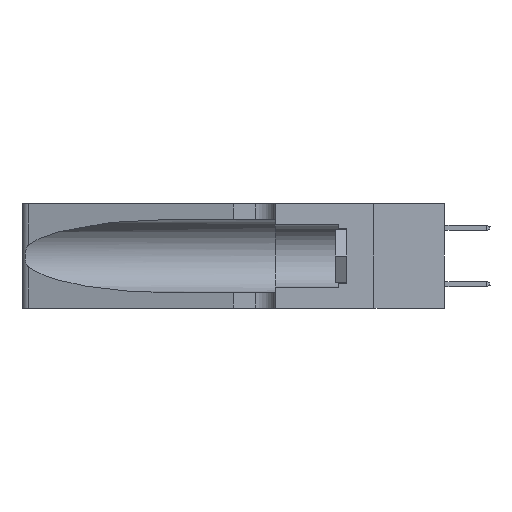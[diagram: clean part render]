
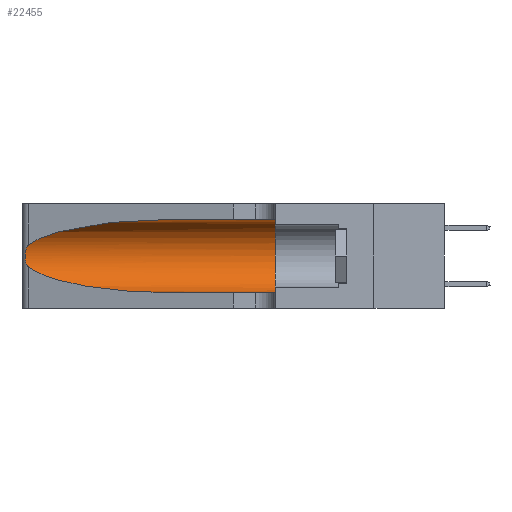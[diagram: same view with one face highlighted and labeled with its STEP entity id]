
A CAD part, left-side view. The second image highlights one B-rep face of the part: STEP entity #22455.
In plain terms, the highlighted cylindrical face has radius 3.308 mm (diameter 6.617 mm), a partial arc.
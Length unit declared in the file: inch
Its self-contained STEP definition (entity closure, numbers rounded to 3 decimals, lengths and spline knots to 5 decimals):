
#5 = LINE ( 'NONE', #20721, #28633 ) ;
#314 = CARTESIAN_POINT ( 'NONE',  ( 0.1305, 0.35, 0.185 ) ) ;
#652 = CARTESIAN_POINT ( 'NONE',  ( 0.25555, 1.22994, 0.2215 ) ) ;
#765 = CARTESIAN_POINT ( 'NONE',  ( 0.25639, 1.23186, 0.15144 ) ) ;
#859 = ORIENTED_EDGE ( 'NONE', *, *, #6011, .F. ) ;
#998 = CARTESIAN_POINT ( 'NONE',  ( 0.25487, 1.22718, 0.22369 ) ) ;
#1341 = CARTESIAN_POINT ( 'NONE',  ( 0.25487, 1.22718, 0.14631 ) ) ;
#1669 = EDGE_CURVE ( 'NONE', #19165, #28585, #19838, .T. ) ;
#1721 = EDGE_CURVE ( 'NONE', #27023, #28585, #18414, .T. ) ;
#2935 = CARTESIAN_POINT ( 'NONE',  ( 0.25487, 1.22718, 0.22369 ) ) ;
#3111 = CARTESIAN_POINT ( 'NONE',  ( 0.25487, 1.22718, 0.14631 ) ) ;
#3691 = CARTESIAN_POINT ( 'NONE',  ( 0.1305, 0.72297, 0.05475 ) ) ;
#3912 = DIRECTION ( 'NONE',  ( 0., 0., 1. ) ) ;
#4054 = CARTESIAN_POINT ( 'NONE',  ( 0.1305, 0.35, 0.31525 ) ) ;
#5382 = CARTESIAN_POINT ( 'NONE',  ( 0.25639, 1.23184, 0.21858 ) ) ;
#5555 = CARTESIAN_POINT ( 'NONE',  ( 0.1305, 0.72297, 0.31525 ) ) ;
#6011 = EDGE_CURVE ( 'NONE', #16149, #27023, #5, .T. ) ;
#7574 = VECTOR ( 'NONE', #9677, 39.37008 ) ;
#7730 = CARTESIAN_POINT ( 'NONE',  ( 0.25854, 1.2359, 0.20912 ) ) ;
#8211 = CARTESIAN_POINT ( 'NONE',  ( 0.2373, 1.15595, 0.08982 ) ) ;
#8571 = CARTESIAN_POINT ( 'NONE',  ( 0.25487, 1.22718, 0.14631 ) ) ;
#9151 = DIRECTION ( 'NONE',  ( 0., 0., -1. ) ) ;
#9458 = EDGE_LOOP ( 'NONE', ( #29984, #18600, #20854, #19715, #18044, #859 ) ) ;
#9677 = DIRECTION ( 'NONE',  ( 0., -1., 0. ) ) ;
#9701 = AXIS2_PLACEMENT_3D ( 'NONE', #25240, #27578, #9151 ) ;
#9716 = CARTESIAN_POINT ( 'NONE',  ( 0.1305, 0.35, 0.05475 ) ) ;
#10058 = CARTESIAN_POINT ( 'NONE',  ( 0.26075, 1.23896, 0.19203 ) ) ;
#12350 = CARTESIAN_POINT ( 'NONE',  ( 0.26017, 1.23833, 0.17102 ) ) ;
#13036 = B_SPLINE_CURVE_WITH_KNOTS ( 'NONE', 3,
 ( #16907, #652, #5382, #21539, #7730, #23842, #10058, #26157, #12350, #28484, #14704, #765, #16997, #3111 ),
 .UNSPECIFIED., .F., .F.,
 ( 4, 2, 2, 2, 2, 2, 4 ),
 ( 0., 0.00027, 0.00053, 0.00107, 0.0016, 0.00187, 0.00214 ),
 .UNSPECIFIED. ) ;
#13652 =( BOUNDED_CURVE ( )  B_SPLINE_CURVE ( 3, ( #14940, #26372, #21768, #998 ),
 .UNSPECIFIED., .F., .T. ) 
 B_SPLINE_CURVE_WITH_KNOTS ( ( 4, 4 ),
 ( 1.5708, 2.84003 ),
 .UNSPECIFIED. ) 
 CURVE ( )  GEOMETRIC_REPRESENTATION_ITEM ( )  RATIONAL_B_SPLINE_CURVE ( ( 1., 0.87, 0.87, 1. ) ) 
 REPRESENTATION_ITEM ( '' )  );
#13941 = AXIS2_PLACEMENT_3D ( 'NONE', #314, #21217, #3912 ) ;
#14704 = CARTESIAN_POINT ( 'NONE',  ( 0.25789, 1.23486, 0.15765 ) ) ;
#14940 = CARTESIAN_POINT ( 'NONE',  ( 0.1305, 0.72297, 0.31525 ) ) ;
#14952 = EDGE_CURVE ( 'NONE', #16149, #16746, #13652, .T. ) ;
#16149 = VERTEX_POINT ( 'NONE', #5555 ) ;
#16746 = VERTEX_POINT ( 'NONE', #2935 ) ;
#16907 = CARTESIAN_POINT ( 'NONE',  ( 0.25487, 1.22718, 0.22369 ) ) ;
#16997 = CARTESIAN_POINT ( 'NONE',  ( 0.25555, 1.22993, 0.14849 ) ) ;
#18044 = ORIENTED_EDGE ( 'NONE', *, *, #1721, .F. ) ;
#18301 = EDGE_CURVE ( 'NONE', #25208, #19165, #21748, .T. ) ;
#18414 = CIRCLE ( 'NONE', #13941, 0.13025 ) ;
#18571 = CARTESIAN_POINT ( 'NONE',  ( 0.1305, 0.72297, 0.05475 ) ) ;
#18600 = ORIENTED_EDGE ( 'NONE', *, *, #27414, .T. ) ;
#19165 = VERTEX_POINT ( 'NONE', #18571 ) ;
#19715 = ORIENTED_EDGE ( 'NONE', *, *, #1669, .T. ) ;
#19838 = LINE ( 'NONE', #23276, #7574 ) ;
#20721 = CARTESIAN_POINT ( 'NONE',  ( 0.1305, 1.61858, 0.31525 ) ) ;
#20854 = ORIENTED_EDGE ( 'NONE', *, *, #18301, .T. ) ;
#21217 = DIRECTION ( 'NONE',  ( 0., 1., 0. ) ) ;
#21539 = CARTESIAN_POINT ( 'NONE',  ( 0.25787, 1.23484, 0.2124 ) ) ;
#21748 =( BOUNDED_CURVE ( )  B_SPLINE_CURVE ( 3, ( #1341, #8211, #26719, #3691 ),
 .UNSPECIFIED., .F., .T. ) 
 B_SPLINE_CURVE_WITH_KNOTS ( ( 4, 4 ),
 ( 3.44316, 4.71239 ),
 .UNSPECIFIED. ) 
 CURVE ( )  GEOMETRIC_REPRESENTATION_ITEM ( )  RATIONAL_B_SPLINE_CURVE ( ( 1., 0.87, 0.87, 1. ) ) 
 REPRESENTATION_ITEM ( '' )  );
#21768 = CARTESIAN_POINT ( 'NONE',  ( 0.2373, 1.15595, 0.28018 ) ) ;
#22455 = ADVANCED_FACE ( 'NONE', ( #27622 ), #26875, .F. ) ;
#23276 = CARTESIAN_POINT ( 'NONE',  ( 0.1305, 1.61858, 0.05475 ) ) ;
#23842 = CARTESIAN_POINT ( 'NONE',  ( 0.26018, 1.23835, 0.19895 ) ) ;
#25208 = VERTEX_POINT ( 'NONE', #8571 ) ;
#25240 = CARTESIAN_POINT ( 'NONE',  ( 0.1305, 1.61858, 0.185 ) ) ;
#26157 = CARTESIAN_POINT ( 'NONE',  ( 0.26075, 1.23896, 0.178 ) ) ;
#26372 = CARTESIAN_POINT ( 'NONE',  ( 0.18966, 0.96281, 0.31525 ) ) ;
#26719 = CARTESIAN_POINT ( 'NONE',  ( 0.18966, 0.96281, 0.05475 ) ) ;
#26875 = CYLINDRICAL_SURFACE ( 'NONE', #9701, 0.13025 ) ;
#27023 = VERTEX_POINT ( 'NONE', #4054 ) ;
#27414 = EDGE_CURVE ( 'NONE', #16746, #25208, #13036, .T. ) ;
#27578 = DIRECTION ( 'NONE',  ( 0., -1., 0. ) ) ;
#27622 = FACE_OUTER_BOUND ( 'NONE', #9458, .T. ) ;
#27671 = DIRECTION ( 'NONE',  ( 0., -1., 0. ) ) ;
#28484 = CARTESIAN_POINT ( 'NONE',  ( 0.25856, 1.23593, 0.16098 ) ) ;
#28585 = VERTEX_POINT ( 'NONE', #9716 ) ;
#28633 = VECTOR ( 'NONE', #27671, 39.37008 ) ;
#29984 = ORIENTED_EDGE ( 'NONE', *, *, #14952, .T. ) ;
